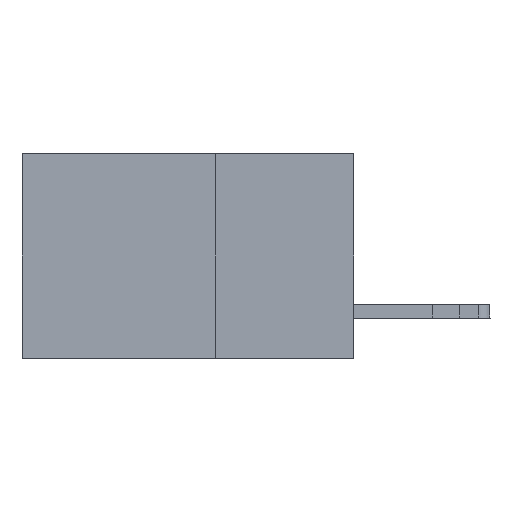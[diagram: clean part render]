
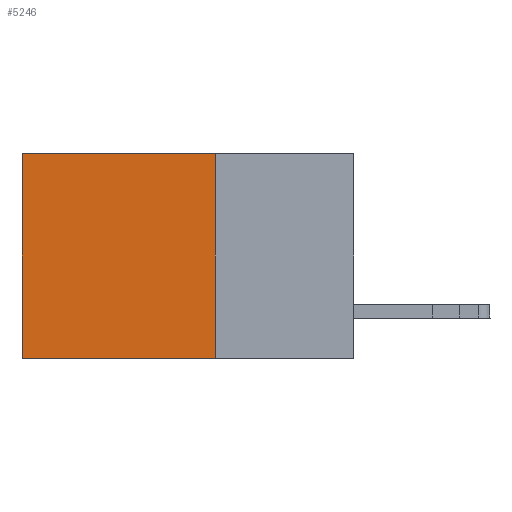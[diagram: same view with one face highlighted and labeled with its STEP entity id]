
A CAD part, left-side view. The second image highlights one B-rep face of the part: STEP entity #5246.
In plain terms, the highlighted planar face has unit normal (-1, 0, 0).
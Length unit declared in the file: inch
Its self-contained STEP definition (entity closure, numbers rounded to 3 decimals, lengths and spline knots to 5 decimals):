
#259 = LINE ( 'NONE', #21348, #2718 ) ;
#481 = CARTESIAN_POINT ( 'NONE',  ( 0.2875, 0.25, -0.37 ) ) ;
#1271 = VERTEX_POINT ( 'NONE', #481 ) ;
#2718 = VECTOR ( 'NONE', #6844, 39.37008 ) ;
#3875 = EDGE_CURVE ( 'NONE', #1271, #9565, #24074, .T. ) ;
#4264 = VERTEX_POINT ( 'NONE', #4945 ) ;
#4874 = DIRECTION ( 'NONE',  ( 0., 0., -1. ) ) ;
#4945 = CARTESIAN_POINT ( 'NONE',  ( 0.2875, 0.6, 0. ) ) ;
#5246 = ADVANCED_FACE ( 'NONE', ( #8625 ), #30376, .F. ) ;
#6766 = CARTESIAN_POINT ( 'NONE',  ( 0.2875, 0.25, 0. ) ) ;
#6844 = DIRECTION ( 'NONE',  ( 0., 0., -1. ) ) ;
#8625 = FACE_OUTER_BOUND ( 'NONE', #9174, .T. ) ;
#9031 = DIRECTION ( 'NONE',  ( 0., 1., 0. ) ) ;
#9174 = EDGE_LOOP ( 'NONE', ( #9983, #17783, #20011, #30720 ) ) ;
#9260 = CARTESIAN_POINT ( 'NONE',  ( 0.2875, 0.25, -0.37 ) ) ;
#9565 = VERTEX_POINT ( 'NONE', #14364 ) ;
#9983 = ORIENTED_EDGE ( 'NONE', *, *, #25375, .T. ) ;
#10427 = DIRECTION ( 'NONE',  ( 1., 0., 0. ) ) ;
#10857 = LINE ( 'NONE', #30407, #22579 ) ;
#11102 = VERTEX_POINT ( 'NONE', #18161 ) ;
#11143 = VECTOR ( 'NONE', #9031, 39.37008 ) ;
#12398 = AXIS2_PLACEMENT_3D ( 'NONE', #22621, #10427, #23278 ) ;
#14364 = CARTESIAN_POINT ( 'NONE',  ( 0.2875, 0.6, -0.37 ) ) ;
#17783 = ORIENTED_EDGE ( 'NONE', *, *, #3875, .F. ) ;
#18161 = CARTESIAN_POINT ( 'NONE',  ( 0.2875, 0.25, 0. ) ) ;
#19584 = DIRECTION ( 'NONE',  ( 0., 1., 0. ) ) ;
#20011 = ORIENTED_EDGE ( 'NONE', *, *, #26937, .F. ) ;
#21348 = CARTESIAN_POINT ( 'NONE',  ( 0.2875, 0.25, 0. ) ) ;
#22579 = VECTOR ( 'NONE', #4874, 39.37008 ) ;
#22621 = CARTESIAN_POINT ( 'NONE',  ( 0.2875, 0.25, 0. ) ) ;
#22811 = VECTOR ( 'NONE', #19584, 39.37008 ) ;
#23180 = LINE ( 'NONE', #6766, #22811 ) ;
#23278 = DIRECTION ( 'NONE',  ( 0., 0., -1. ) ) ;
#24074 = LINE ( 'NONE', #9260, #11143 ) ;
#25375 = EDGE_CURVE ( 'NONE', #4264, #9565, #10857, .T. ) ;
#26937 = EDGE_CURVE ( 'NONE', #11102, #1271, #259, .T. ) ;
#30376 = PLANE ( 'NONE',  #12398 ) ;
#30407 = CARTESIAN_POINT ( 'NONE',  ( 0.2875, 0.6, 0. ) ) ;
#30720 = ORIENTED_EDGE ( 'NONE', *, *, #33323, .T. ) ;
#33323 = EDGE_CURVE ( 'NONE', #11102, #4264, #23180, .T. ) ;
